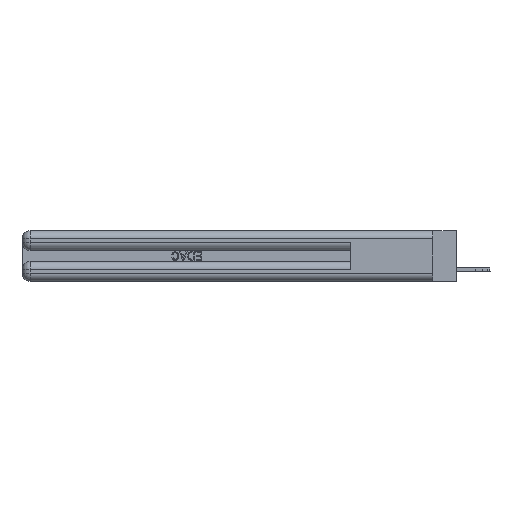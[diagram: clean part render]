
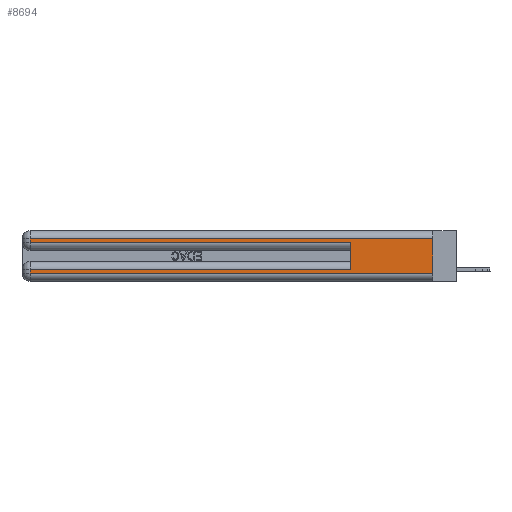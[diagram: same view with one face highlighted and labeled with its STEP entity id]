
A CAD part, left-side view. The second image highlights one B-rep face of the part: STEP entity #8694.
In plain terms, the highlighted planar face has unit normal (-1, 0, 0).
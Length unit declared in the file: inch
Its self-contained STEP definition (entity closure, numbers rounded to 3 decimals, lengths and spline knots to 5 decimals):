
#1329 = FACE_OUTER_BOUND ( 'NONE', #34101, .T. ) ;
#1337 = CARTESIAN_POINT ( 'NONE',  ( 0., 0., 0.37 ) ) ;
#1560 = LINE ( 'NONE', #20742, #32770 ) ;
#1665 = CARTESIAN_POINT ( 'NONE',  ( 0., 2.94, 0.285 ) ) ;
#2213 = LINE ( 'NONE', #18953, #18749 ) ;
#4724 = EDGE_CURVE ( 'NONE', #32264, #13194, #24620, .T. ) ;
#5156 = VECTOR ( 'NONE', #13156, 39.37008 ) ;
#6362 = LINE ( 'NONE', #10097, #35755 ) ;
#7078 = ORIENTED_EDGE ( 'NONE', *, *, #26557, .F. ) ;
#7754 = DIRECTION ( 'NONE',  ( 0., 0., -1. ) ) ;
#8073 = VERTEX_POINT ( 'NONE', #36839 ) ;
#8234 = VERTEX_POINT ( 'NONE', #35251 ) ;
#8694 = ADVANCED_FACE ( 'NONE', ( #1329 ), #15172, .F. ) ;
#10097 = CARTESIAN_POINT ( 'NONE',  ( 0., 0., 0.085 ) ) ;
#13062 = ORIENTED_EDGE ( 'NONE', *, *, #4724, .T. ) ;
#13156 = DIRECTION ( 'NONE',  ( 0., 0., -1. ) ) ;
#13194 = VERTEX_POINT ( 'NONE', #32935 ) ;
#14072 = VERTEX_POINT ( 'NONE', #34896 ) ;
#14522 = VECTOR ( 'NONE', #18747, 39.37008 ) ;
#14719 = ORIENTED_EDGE ( 'NONE', *, *, #23755, .T. ) ;
#14979 = VECTOR ( 'NONE', #28675, 39.37008 ) ;
#15172 = PLANE ( 'NONE',  #26725 ) ;
#15368 = CARTESIAN_POINT ( 'NONE',  ( 0., 0., 0.31 ) ) ;
#15601 = DIRECTION ( 'NONE',  ( 0., -1., 0. ) ) ;
#16852 = EDGE_CURVE ( 'NONE', #23793, #34917, #33624, .T. ) ;
#18167 = ORIENTED_EDGE ( 'NONE', *, *, #24694, .T. ) ;
#18203 = LINE ( 'NONE', #15368, #14522 ) ;
#18576 = CARTESIAN_POINT ( 'NONE',  ( 0., 0., 0.285 ) ) ;
#18747 = DIRECTION ( 'NONE',  ( 0., 1., 0. ) ) ;
#18749 = VECTOR ( 'NONE', #7754, 39.37008 ) ;
#18953 = CARTESIAN_POINT ( 'NONE',  ( 0., 2.94, 0.37 ) ) ;
#20528 = ORIENTED_EDGE ( 'NONE', *, *, #22886, .T. ) ;
#20742 = CARTESIAN_POINT ( 'NONE',  ( 0., 0., 0.06 ) ) ;
#21396 = ORIENTED_EDGE ( 'NONE', *, *, #31031, .T. ) ;
#22737 = ORIENTED_EDGE ( 'NONE', *, *, #16852, .T. ) ;
#22886 = EDGE_CURVE ( 'NONE', #14072, #23793, #2213, .T. ) ;
#22913 = ORIENTED_EDGE ( 'NONE', *, *, #25233, .F. ) ;
#23755 = EDGE_CURVE ( 'NONE', #8234, #14072, #18203, .T. ) ;
#23793 = VERTEX_POINT ( 'NONE', #1665 ) ;
#24354 = CARTESIAN_POINT ( 'NONE',  ( 0., 2.94, 0.085 ) ) ;
#24620 = LINE ( 'NONE', #25665, #14979 ) ;
#24694 = EDGE_CURVE ( 'NONE', #13194, #8073, #1560, .T. ) ;
#25233 = EDGE_CURVE ( 'NONE', #8234, #8073, #36401, .T. ) ;
#25665 = CARTESIAN_POINT ( 'NONE',  ( 0., 2.94, 0.37 ) ) ;
#25971 = VERTEX_POINT ( 'NONE', #26798 ) ;
#26557 = EDGE_CURVE ( 'NONE', #25971, #34917, #30302, .T. ) ;
#26598 = DIRECTION ( 'NONE',  ( 0., -1., 0. ) ) ;
#26725 = AXIS2_PLACEMENT_3D ( 'NONE', #34200, #36785, #37192 ) ;
#26798 = CARTESIAN_POINT ( 'NONE',  ( 0., 0.6, 0.085 ) ) ;
#28014 = VECTOR ( 'NONE', #37784, 39.37008 ) ;
#28675 = DIRECTION ( 'NONE',  ( 0., 0., -1. ) ) ;
#28998 = CARTESIAN_POINT ( 'NONE',  ( 0., 0.6, 0.145 ) ) ;
#30302 = LINE ( 'NONE', #28998, #28014 ) ;
#30674 = DIRECTION ( 'NONE',  ( 0., 1., 0. ) ) ;
#31031 = EDGE_CURVE ( 'NONE', #25971, #32264, #6362, .T. ) ;
#32264 = VERTEX_POINT ( 'NONE', #24354 ) ;
#32770 = VECTOR ( 'NONE', #26598, 39.37008 ) ;
#32935 = CARTESIAN_POINT ( 'NONE',  ( 0., 2.94, 0.06 ) ) ;
#33624 = LINE ( 'NONE', #18576, #34564 ) ;
#34101 = EDGE_LOOP ( 'NONE', ( #22913, #14719, #20528, #22737, #7078, #21396, #13062, #18167 ) ) ;
#34200 = CARTESIAN_POINT ( 'NONE',  ( 0., 0., 0.37 ) ) ;
#34564 = VECTOR ( 'NONE', #15601, 39.37008 ) ;
#34896 = CARTESIAN_POINT ( 'NONE',  ( 0., 2.94, 0.31 ) ) ;
#34917 = VERTEX_POINT ( 'NONE', #37240 ) ;
#35251 = CARTESIAN_POINT ( 'NONE',  ( 0., 0., 0.31 ) ) ;
#35755 = VECTOR ( 'NONE', #30674, 39.37008 ) ;
#36401 = LINE ( 'NONE', #1337, #5156 ) ;
#36785 = DIRECTION ( 'NONE',  ( 1., 0., 0. ) ) ;
#36839 = CARTESIAN_POINT ( 'NONE',  ( 0., 0., 0.06 ) ) ;
#37192 = DIRECTION ( 'NONE',  ( 0., 0., -1. ) ) ;
#37240 = CARTESIAN_POINT ( 'NONE',  ( 0., 0.6, 0.285 ) ) ;
#37784 = DIRECTION ( 'NONE',  ( 0., 0., 1. ) ) ;
